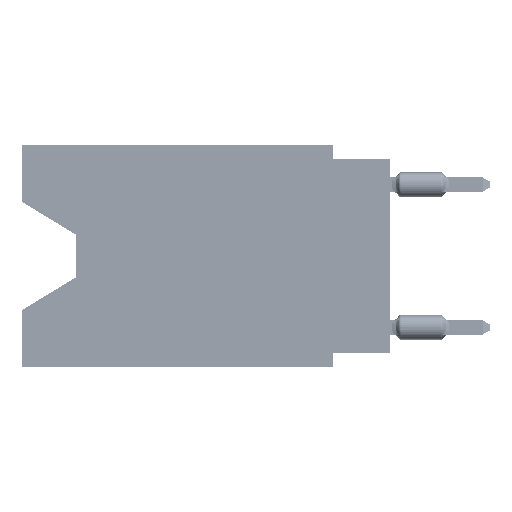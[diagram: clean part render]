
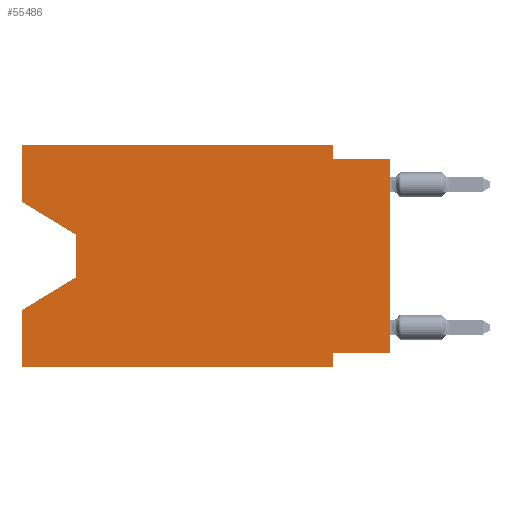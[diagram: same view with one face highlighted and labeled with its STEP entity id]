
A CAD part, left-side view. The second image highlights one B-rep face of the part: STEP entity #55486.
In plain terms, the highlighted planar face has unit normal (-1, 0, 0).
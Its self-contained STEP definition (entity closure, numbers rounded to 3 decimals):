
#981 = EDGE_CURVE ( 'NONE', #47156, #60993, #31947, .T. ) ;
#2225 = ORIENTED_EDGE ( 'NONE', *, *, #981, .T. ) ;
#2906 = DIRECTION ( 'NONE',  ( 0., 0., -1. ) ) ;
#3127 = DIRECTION ( 'NONE',  ( 0., 0., -1. ) ) ;
#4738 = EDGE_LOOP ( 'NONE', ( #61469, #69492, #23903, #51802, #2225, #58020, #9477, #33056, #57467, #31412, #20358, #47021 ) ) ;
#5439 = VERTEX_POINT ( 'NONE', #24065 ) ;
#5929 = CARTESIAN_POINT ( 'NONE',  ( 0., 2.54, -9.906 ) ) ;
#6174 = EDGE_CURVE ( 'NONE', #16499, #25480, #15692, .T. ) ;
#6739 = EDGE_CURVE ( 'NONE', #25054, #11939, #44413, .T. ) ;
#6938 = VERTEX_POINT ( 'NONE', #22818 ) ;
#8007 = DIRECTION ( 'NONE',  ( 0., 0., 1. ) ) ;
#8415 = DIRECTION ( 'NONE',  ( 0., 0., -1. ) ) ;
#9178 = VECTOR ( 'NONE', #42431, 1000. ) ;
#9477 = ORIENTED_EDGE ( 'NONE', *, *, #6739, .F. ) ;
#9989 = LINE ( 'NONE', #75792, #44698 ) ;
#10653 = CARTESIAN_POINT ( 'NONE',  ( 0., 16.383, -9.906 ) ) ;
#11939 = VERTEX_POINT ( 'NONE', #54637 ) ;
#12838 = EDGE_CURVE ( 'NONE', #47156, #51332, #69256, .T. ) ;
#15692 = LINE ( 'NONE', #57616, #54722 ) ;
#16088 = CARTESIAN_POINT ( 'NONE',  ( 0., 2.54, 0. ) ) ;
#16499 = VERTEX_POINT ( 'NONE', #39208 ) ;
#16809 = VECTOR ( 'NONE', #74744, 1000. ) ;
#18512 = CARTESIAN_POINT ( 'NONE',  ( 0., 0., 0. ) ) ;
#19247 = VECTOR ( 'NONE', #55860, 1000. ) ;
#19469 = CARTESIAN_POINT ( 'NONE',  ( 0., 13.97, -4.013 ) ) ;
#20358 = ORIENTED_EDGE ( 'NONE', *, *, #36992, .F. ) ;
#22043 = LINE ( 'NONE', #33429, #48563 ) ;
#22064 = EDGE_CURVE ( 'NONE', #16499, #76063, #37813, .T. ) ;
#22818 = CARTESIAN_POINT ( 'NONE',  ( 0., 2.54, -0.635 ) ) ;
#23903 = ORIENTED_EDGE ( 'NONE', *, *, #53747, .T. ) ;
#24065 = CARTESIAN_POINT ( 'NONE',  ( 0., 2.54, 0. ) ) ;
#25054 = VERTEX_POINT ( 'NONE', #43880 ) ;
#25480 = VERTEX_POINT ( 'NONE', #19469 ) ;
#25851 = EDGE_CURVE ( 'NONE', #25054, #48280, #72169, .T. ) ;
#27460 = LINE ( 'NONE', #16088, #61602 ) ;
#27625 = LINE ( 'NONE', #38605, #52709 ) ;
#27829 = DIRECTION ( 'NONE',  ( 0., -0.855, -0.519 ) ) ;
#27928 = DIRECTION ( 'NONE',  ( 0., 0., -1. ) ) ;
#31412 = ORIENTED_EDGE ( 'NONE', *, *, #47682, .F. ) ;
#31947 = LINE ( 'NONE', #49982, #19247 ) ;
#32237 = CARTESIAN_POINT ( 'NONE',  ( 0., 16.383, 0. ) ) ;
#32318 = CARTESIAN_POINT ( 'NONE',  ( 0., 16.383, 0. ) ) ;
#33056 = ORIENTED_EDGE ( 'NONE', *, *, #25851, .T. ) ;
#33429 = CARTESIAN_POINT ( 'NONE',  ( 0., 13.97, -4.013 ) ) ;
#34401 = CARTESIAN_POINT ( 'NONE',  ( 0., 16.383, 0. ) ) ;
#34442 = CARTESIAN_POINT ( 'NONE',  ( 0., 16.383, 0. ) ) ;
#34662 = DIRECTION ( 'NONE',  ( 0., -1., 0. ) ) ;
#34811 = AXIS2_PLACEMENT_3D ( 'NONE', #50734, #49589, #8415 ) ;
#34888 = EDGE_CURVE ( 'NONE', #11939, #60993, #27625, .T. ) ;
#35603 = LINE ( 'NONE', #54784, #77465 ) ;
#36064 = CARTESIAN_POINT ( 'NONE',  ( 0., 13.97, -5.893 ) ) ;
#36992 = EDGE_CURVE ( 'NONE', #76063, #5439, #69026, .T. ) ;
#37813 = LINE ( 'NONE', #32318, #61365 ) ;
#38605 = CARTESIAN_POINT ( 'NONE',  ( 0., 2.54, -9.906 ) ) ;
#39208 = CARTESIAN_POINT ( 'NONE',  ( 0., 16.383, -2.546 ) ) ;
#42431 = DIRECTION ( 'NONE',  ( 0., 0., 1. ) ) ;
#43505 = CARTESIAN_POINT ( 'NONE',  ( 0., 0., -0.635 ) ) ;
#43880 = CARTESIAN_POINT ( 'NONE',  ( 0., 0., -9.271 ) ) ;
#44413 = LINE ( 'NONE', #50290, #51032 ) ;
#44698 = VECTOR ( 'NONE', #34662, 1000. ) ;
#47021 = ORIENTED_EDGE ( 'NONE', *, *, #22064, .F. ) ;
#47156 = VERTEX_POINT ( 'NONE', #10653 ) ;
#47682 = EDGE_CURVE ( 'NONE', #5439, #6938, #27460, .T. ) ;
#48280 = VERTEX_POINT ( 'NONE', #43505 ) ;
#48563 = VECTOR ( 'NONE', #27928, 1000. ) ;
#49589 = DIRECTION ( 'NONE',  ( 1., 0., 0. ) ) ;
#49982 = CARTESIAN_POINT ( 'NONE',  ( 0., 16.383, -9.906 ) ) ;
#50254 = DIRECTION ( 'NONE',  ( 0., -1., 0. ) ) ;
#50290 = CARTESIAN_POINT ( 'NONE',  ( 0., 0., -9.271 ) ) ;
#50734 = CARTESIAN_POINT ( 'NONE',  ( 0., 16.383, 0. ) ) ;
#51032 = VECTOR ( 'NONE', #74948, 1000. ) ;
#51332 = VERTEX_POINT ( 'NONE', #76084 ) ;
#51611 = EDGE_CURVE ( 'NONE', #6938, #48280, #9989, .T. ) ;
#51802 = ORIENTED_EDGE ( 'NONE', *, *, #12838, .F. ) ;
#52709 = VECTOR ( 'NONE', #2906, 1000. ) ;
#53747 = EDGE_CURVE ( 'NONE', #75032, #51332, #35603, .T. ) ;
#54637 = CARTESIAN_POINT ( 'NONE',  ( 0., 2.54, -9.271 ) ) ;
#54722 = VECTOR ( 'NONE', #27829, 1000. ) ;
#54784 = CARTESIAN_POINT ( 'NONE',  ( 0., 13.97, -5.893 ) ) ;
#55470 = PLANE ( 'NONE',  #34811 ) ;
#55486 = ADVANCED_FACE ( 'NONE', ( #62090 ), #55470, .F. ) ;
#55860 = DIRECTION ( 'NONE',  ( 0., -1., 0. ) ) ;
#56812 = EDGE_CURVE ( 'NONE', #25480, #75032, #22043, .T. ) ;
#57467 = ORIENTED_EDGE ( 'NONE', *, *, #51611, .F. ) ;
#57616 = CARTESIAN_POINT ( 'NONE',  ( 0., 16.383, -2.546 ) ) ;
#58020 = ORIENTED_EDGE ( 'NONE', *, *, #34888, .F. ) ;
#60993 = VERTEX_POINT ( 'NONE', #5929 ) ;
#61365 = VECTOR ( 'NONE', #8007, 1000. ) ;
#61469 = ORIENTED_EDGE ( 'NONE', *, *, #6174, .T. ) ;
#61602 = VECTOR ( 'NONE', #3127, 1000. ) ;
#62090 = FACE_OUTER_BOUND ( 'NONE', #4738, .T. ) ;
#62860 = VECTOR ( 'NONE', #50254, 1000. ) ;
#66131 = DIRECTION ( 'NONE',  ( 0., 0.855, -0.519 ) ) ;
#69026 = LINE ( 'NONE', #32237, #62860 ) ;
#69256 = LINE ( 'NONE', #34401, #16809 ) ;
#69492 = ORIENTED_EDGE ( 'NONE', *, *, #56812, .T. ) ;
#72169 = LINE ( 'NONE', #18512, #9178 ) ;
#74744 = DIRECTION ( 'NONE',  ( 0., 0., 1. ) ) ;
#74948 = DIRECTION ( 'NONE',  ( 0., 1., 0. ) ) ;
#75032 = VERTEX_POINT ( 'NONE', #36064 ) ;
#75792 = CARTESIAN_POINT ( 'NONE',  ( 0., 0., -0.635 ) ) ;
#76063 = VERTEX_POINT ( 'NONE', #34442 ) ;
#76084 = CARTESIAN_POINT ( 'NONE',  ( 0., 16.383, -7.36 ) ) ;
#77465 = VECTOR ( 'NONE', #66131, 1000. ) ;
